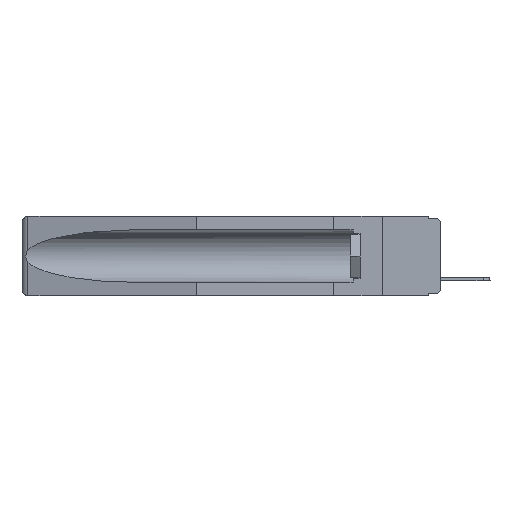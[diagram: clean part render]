
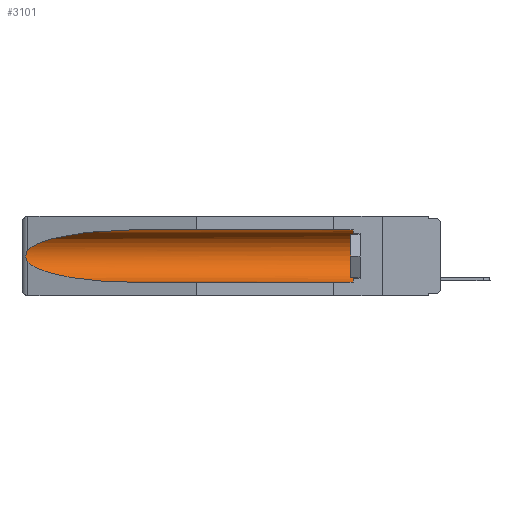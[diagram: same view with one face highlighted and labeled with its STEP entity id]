
A CAD part, left-side view. The second image highlights one B-rep face of the part: STEP entity #3101.
In plain terms, the highlighted cylindrical face has radius 2.857 mm (diameter 5.715 mm), a partial arc.
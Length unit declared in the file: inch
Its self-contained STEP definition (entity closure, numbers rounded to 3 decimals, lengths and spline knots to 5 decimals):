
#25 =( BOUNDED_CURVE ( )  B_SPLINE_CURVE ( 3, ( #1151, #24037, #5130, #22064 ),
 .UNSPECIFIED., .F., .F. ) 
 B_SPLINE_CURVE_WITH_KNOTS ( ( 4, 4 ),
 ( 4.71239, 6.08839 ),
 .UNSPECIFIED. ) 
 CURVE ( )  GEOMETRIC_REPRESENTATION_ITEM ( )  RATIONAL_B_SPLINE_CURVE ( ( 1., 0.848, 0.848, 1. ) ) 
 REPRESENTATION_ITEM ( '' )  );
#997 = CARTESIAN_POINT ( 'NONE',  ( 0.155, -0.30754, -0.1715 ) ) ;
#1151 = CARTESIAN_POINT ( 'NONE',  ( 0.155, 1.07973, -0.059 ) ) ;
#1395 = CARTESIAN_POINT ( 'NONE',  ( 0.26537, 1.52718, -0.14972 ) ) ;
#2706 = EDGE_CURVE ( 'NONE', #2959, #19533, #25, .T. ) ;
#2959 = VERTEX_POINT ( 'NONE', #9845 ) ;
#3101 = ADVANCED_FACE ( 'NONE', ( #24003 ), #10576, .F. ) ;
#3379 = ORIENTED_EDGE ( 'NONE', *, *, #11170, .T. ) ;
#3392 = CARTESIAN_POINT ( 'NONE',  ( 0.2675, 1.53308, -0.16763 ) ) ;
#3480 = DIRECTION ( 'NONE',  ( 0., -1., 0. ) ) ;
#4381 = ORIENTED_EDGE ( 'NONE', *, *, #20216, .F. ) ;
#4899 = CARTESIAN_POINT ( 'NONE',  ( 0.26537, 1.52718, -0.19328 ) ) ;
#5130 = CARTESIAN_POINT ( 'NONE',  ( 0.25451, 1.48313, -0.09465 ) ) ;
#5226 = VECTOR ( 'NONE', #16320, 39.37008 ) ;
#5232 = CARTESIAN_POINT ( 'NONE',  ( 0.26537, 1.52718, -0.19328 ) ) ;
#5377 = CARTESIAN_POINT ( 'NONE',  ( 0.2673, 1.5327, -0.16383 ) ) ;
#5497 = CARTESIAN_POINT ( 'NONE',  ( 0.26537, 1.52718, -0.19328 ) ) ;
#5614 = CARTESIAN_POINT ( 'NONE',  ( 0.26655, 1.53094, -0.18657 ) ) ;
#5783 = EDGE_CURVE ( 'NONE', #10736, #15217, #7668, .T. ) ;
#6642 = LINE ( 'NONE', #10484, #5226 ) ;
#6766 = VECTOR ( 'NONE', #17056, 39.37008 ) ;
#6850 = DIRECTION ( 'NONE',  ( 0., 1., 0. ) ) ;
#7382 = ORIENTED_EDGE ( 'NONE', *, *, #9662, .T. ) ;
#7668 =( BOUNDED_CURVE ( )  B_SPLINE_CURVE ( 3, ( #5232, #10329, #12320, #16046 ),
 .UNSPECIFIED., .F., .F. ) 
 B_SPLINE_CURVE_WITH_KNOTS ( ( 4, 4 ),
 ( 0.1948, 1.5708 ),
 .UNSPECIFIED. ) 
 CURVE ( )  GEOMETRIC_REPRESENTATION_ITEM ( )  RATIONAL_B_SPLINE_CURVE ( ( 1., 0.848, 0.848, 1. ) ) 
 REPRESENTATION_ITEM ( '' )  );
#8457 = ORIENTED_EDGE ( 'NONE', *, *, #12611, .T. ) ;
#8766 = ORIENTED_EDGE ( 'NONE', *, *, #2706, .T. ) ;
#9599 = CARTESIAN_POINT ( 'NONE',  ( 0.155, -0.30754, -0.059 ) ) ;
#9662 = EDGE_CURVE ( 'NONE', #12401, #2959, #22790, .T. ) ;
#9845 = CARTESIAN_POINT ( 'NONE',  ( 0.155, 1.07973, -0.059 ) ) ;
#10329 = CARTESIAN_POINT ( 'NONE',  ( 0.25451, 1.48313, -0.24835 ) ) ;
#10484 = CARTESIAN_POINT ( 'NONE',  ( 0.155, -0.30754, -0.284 ) ) ;
#10576 = CYLINDRICAL_SURFACE ( 'NONE', #15208, 0.1125 ) ;
#10695 = CARTESIAN_POINT ( 'NONE',  ( 0.155, 0.126, -0.284 ) ) ;
#10736 = VERTEX_POINT ( 'NONE', #4899 ) ;
#11170 = EDGE_CURVE ( 'NONE', #20517, #12401, #15540, .T. ) ;
#11350 = CARTESIAN_POINT ( 'NONE',  ( 0.2675, 1.53308, -0.17534 ) ) ;
#11726 = B_SPLINE_CURVE_WITH_KNOTS ( 'NONE', 3,
 ( #1395, #20793, #24263, #5377, #3392, #11350, #14949, #5614, #12833, #5497 ),
 .UNSPECIFIED., .F., .F.,
 ( 4, 2, 2, 2, 4 ),
 ( 0., 0.00029, 0.00058, 0.00087, 0.00117 ),
 .UNSPECIFIED. ) ;
#12320 = CARTESIAN_POINT ( 'NONE',  ( 0.21114, 1.30732, -0.284 ) ) ;
#12401 = VERTEX_POINT ( 'NONE', #19569 ) ;
#12611 = EDGE_CURVE ( 'NONE', #19533, #10736, #11726, .T. ) ;
#12833 = CARTESIAN_POINT ( 'NONE',  ( 0.26597, 1.5296, -0.19026 ) ) ;
#14421 = DIRECTION ( 'NONE',  ( 0., 0., 1. ) ) ;
#14782 = CARTESIAN_POINT ( 'NONE',  ( 0.155, 0.126, -0.1715 ) ) ;
#14949 = CARTESIAN_POINT ( 'NONE',  ( 0.2673, 1.53269, -0.17917 ) ) ;
#15208 = AXIS2_PLACEMENT_3D ( 'NONE', #997, #6850, #14421 ) ;
#15217 = VERTEX_POINT ( 'NONE', #18617 ) ;
#15540 = CIRCLE ( 'NONE', #16759, 0.1125 ) ;
#15840 = ORIENTED_EDGE ( 'NONE', *, *, #5783, .T. ) ;
#16046 = CARTESIAN_POINT ( 'NONE',  ( 0.155, 1.07973, -0.284 ) ) ;
#16320 = DIRECTION ( 'NONE',  ( 0., 1., 0. ) ) ;
#16521 = DIRECTION ( 'NONE',  ( 0., 0., 1. ) ) ;
#16759 = AXIS2_PLACEMENT_3D ( 'NONE', #14782, #3480, #16521 ) ;
#17056 = DIRECTION ( 'NONE',  ( 0., 1., 0. ) ) ;
#18617 = CARTESIAN_POINT ( 'NONE',  ( 0.155, 1.07973, -0.284 ) ) ;
#19533 = VERTEX_POINT ( 'NONE', #23095 ) ;
#19569 = CARTESIAN_POINT ( 'NONE',  ( 0.155, 0.126, -0.059 ) ) ;
#20216 = EDGE_CURVE ( 'NONE', #20517, #15217, #6642, .T. ) ;
#20517 = VERTEX_POINT ( 'NONE', #10695 ) ;
#20793 = CARTESIAN_POINT ( 'NONE',  ( 0.26597, 1.52961, -0.15275 ) ) ;
#21216 = EDGE_LOOP ( 'NONE', ( #8766, #8457, #15840, #4381, #3379, #7382 ) ) ;
#22064 = CARTESIAN_POINT ( 'NONE',  ( 0.26537, 1.52718, -0.14972 ) ) ;
#22790 = LINE ( 'NONE', #9599, #6766 ) ;
#23095 = CARTESIAN_POINT ( 'NONE',  ( 0.26537, 1.52718, -0.14972 ) ) ;
#24003 = FACE_OUTER_BOUND ( 'NONE', #21216, .T. ) ;
#24037 = CARTESIAN_POINT ( 'NONE',  ( 0.21114, 1.30732, -0.059 ) ) ;
#24263 = CARTESIAN_POINT ( 'NONE',  ( 0.26654, 1.53092, -0.15636 ) ) ;
